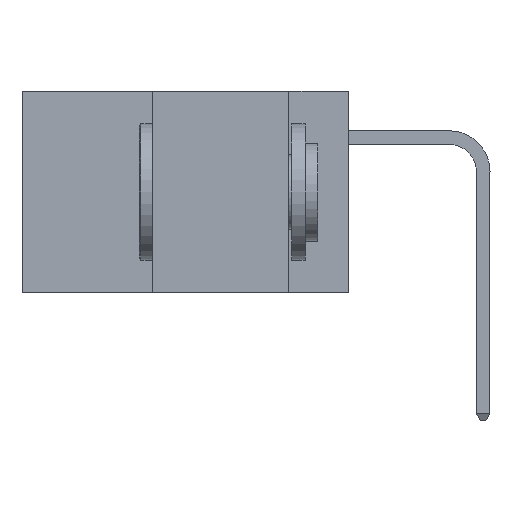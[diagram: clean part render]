
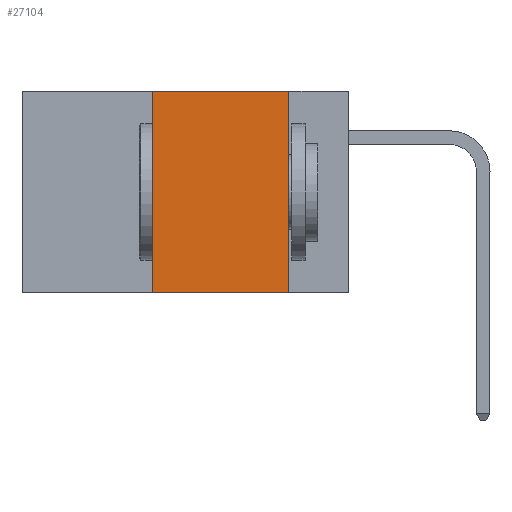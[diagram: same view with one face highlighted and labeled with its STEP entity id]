
A CAD part, left-side view. The second image highlights one B-rep face of the part: STEP entity #27104.
In plain terms, the highlighted planar face has unit normal (-1, 0, 0).
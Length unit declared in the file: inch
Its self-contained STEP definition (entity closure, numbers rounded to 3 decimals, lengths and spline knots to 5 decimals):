
#233 = DIRECTION ( 'NONE',  ( 0., -1., 0. ) ) ;
#1498 = VERTEX_POINT ( 'NONE', #29257 ) ;
#2115 = VERTEX_POINT ( 'NONE', #16147 ) ;
#3226 = EDGE_CURVE ( 'NONE', #16000, #2115, #21863, .T. ) ;
#5602 = CARTESIAN_POINT ( 'NONE',  ( 0., 0.11, -0.37 ) ) ;
#5715 = DIRECTION ( 'NONE',  ( 0., -1., 0. ) ) ;
#5770 = ORIENTED_EDGE ( 'NONE', *, *, #16948, .F. ) ;
#7711 = CARTESIAN_POINT ( 'NONE',  ( 0., 0.6, 0. ) ) ;
#9296 = VECTOR ( 'NONE', #233, 39.37008 ) ;
#10143 = CARTESIAN_POINT ( 'NONE',  ( 0., 0.36, -0.37 ) ) ;
#10285 = DIRECTION ( 'NONE',  ( 0., 0., -1. ) ) ;
#10406 = CARTESIAN_POINT ( 'NONE',  ( 0., 0.6, 0. ) ) ;
#15259 = DIRECTION ( 'NONE',  ( 0., 0., -1. ) ) ;
#15971 = CARTESIAN_POINT ( 'NONE',  ( 0., 0.36, 0. ) ) ;
#16000 = VERTEX_POINT ( 'NONE', #10143 ) ;
#16147 = CARTESIAN_POINT ( 'NONE',  ( 0., 0.36, 0. ) ) ;
#16281 = LINE ( 'NONE', #18363, #17090 ) ;
#16866 = LINE ( 'NONE', #10406, #9296 ) ;
#16948 = EDGE_CURVE ( 'NONE', #2115, #1498, #16866, .T. ) ;
#17090 = VECTOR ( 'NONE', #5715, 39.37008 ) ;
#17530 = EDGE_CURVE ( 'NONE', #1498, #24381, #30868, .T. ) ;
#17850 = PLANE ( 'NONE',  #29655 ) ;
#18363 = CARTESIAN_POINT ( 'NONE',  ( 0., 0.6, -0.37 ) ) ;
#18534 = DIRECTION ( 'NONE',  ( 0., 0., 1. ) ) ;
#18900 = ORIENTED_EDGE ( 'NONE', *, *, #3226, .F. ) ;
#20278 = CARTESIAN_POINT ( 'NONE',  ( 0., 0.11, 0. ) ) ;
#20918 = FACE_OUTER_BOUND ( 'NONE', #24457, .T. ) ;
#21046 = VECTOR ( 'NONE', #18534, 39.37008 ) ;
#21863 = LINE ( 'NONE', #15971, #21046 ) ;
#24011 = VECTOR ( 'NONE', #15259, 39.37008 ) ;
#24381 = VERTEX_POINT ( 'NONE', #5602 ) ;
#24396 = EDGE_CURVE ( 'NONE', #16000, #24381, #16281, .T. ) ;
#24457 = EDGE_LOOP ( 'NONE', ( #30938, #5770, #18900, #27002 ) ) ;
#25588 = DIRECTION ( 'NONE',  ( 1., 0., 0. ) ) ;
#27002 = ORIENTED_EDGE ( 'NONE', *, *, #24396, .T. ) ;
#27104 = ADVANCED_FACE ( 'NONE', ( #20918 ), #17850, .F. ) ;
#29257 = CARTESIAN_POINT ( 'NONE',  ( 0., 0.11, 0. ) ) ;
#29655 = AXIS2_PLACEMENT_3D ( 'NONE', #7711, #25588, #10285 ) ;
#30868 = LINE ( 'NONE', #20278, #24011 ) ;
#30938 = ORIENTED_EDGE ( 'NONE', *, *, #17530, .F. ) ;
